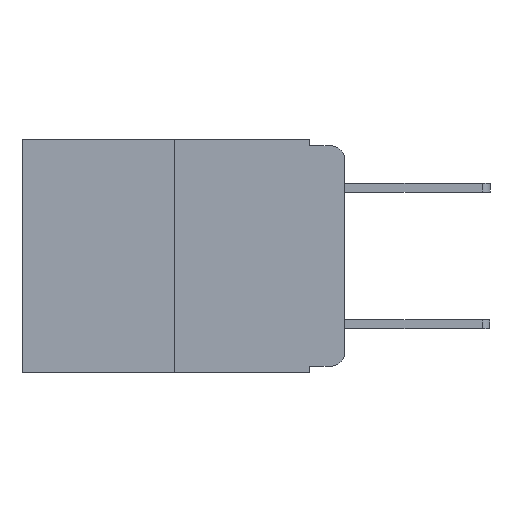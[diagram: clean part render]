
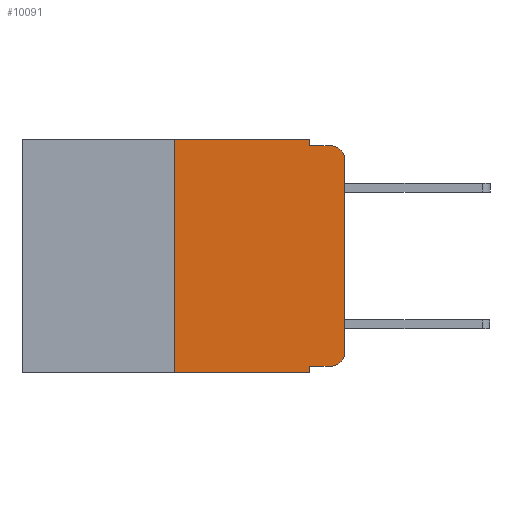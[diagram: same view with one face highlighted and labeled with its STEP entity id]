
A CAD part, left-side view. The second image highlights one B-rep face of the part: STEP entity #10091.
In plain terms, the highlighted planar face has unit normal (-1, 0, 0).
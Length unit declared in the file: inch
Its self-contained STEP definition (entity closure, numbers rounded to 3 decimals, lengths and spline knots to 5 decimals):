
#117 = ORIENTED_EDGE ( 'NONE', *, *, #6094, .T. ) ;
#219 = CARTESIAN_POINT ( 'NONE',  ( 0., 0.473, -0.343 ) ) ;
#726 = EDGE_CURVE ( 'NONE', #4347, #4538, #12148, .T. ) ;
#972 = DIRECTION ( 'NONE',  ( 1., 0., 0. ) ) ;
#1107 = VERTEX_POINT ( 'NONE', #7958 ) ;
#1331 = VERTEX_POINT ( 'NONE', #15850 ) ;
#1384 = DIRECTION ( 'NONE',  ( 0., 0., -1. ) ) ;
#1502 = DIRECTION ( 'NONE',  ( -1., 0., 0. ) ) ;
#1890 = ORIENTED_EDGE ( 'NONE', *, *, #19439, .T. ) ;
#1897 = EDGE_LOOP ( 'NONE', ( #117, #9946, #16369, #5119, #18560, #11007, #1890, #16342, #3068, #16850 ) ) ;
#2301 = VERTEX_POINT ( 'NONE', #17408 ) ;
#2786 = EDGE_CURVE ( 'NONE', #1331, #1107, #20935, .T. ) ;
#2883 = VECTOR ( 'NONE', #16946, 39.37008 ) ;
#3055 = CARTESIAN_POINT ( 'NONE',  ( 0., 0.473, 0. ) ) ;
#3068 = ORIENTED_EDGE ( 'NONE', *, *, #2786, .T. ) ;
#3369 = VECTOR ( 'NONE', #11215, 39.37008 ) ;
#3531 = CARTESIAN_POINT ( 'NONE',  ( 0., 0.02, -0.03 ) ) ;
#3875 = CIRCLE ( 'NONE', #17647, 0.02 ) ;
#4264 = CARTESIAN_POINT ( 'NONE',  ( 0., 0., -0.313 ) ) ;
#4347 = VERTEX_POINT ( 'NONE', #21938 ) ;
#4538 = VERTEX_POINT ( 'NONE', #9941 ) ;
#5119 = ORIENTED_EDGE ( 'NONE', *, *, #13500, .F. ) ;
#5475 = VECTOR ( 'NONE', #10614, 39.37008 ) ;
#5913 = EDGE_CURVE ( 'NONE', #1331, #17348, #18840, .T. ) ;
#6094 = EDGE_CURVE ( 'NONE', #14765, #4347, #20506, .T. ) ;
#6345 = AXIS2_PLACEMENT_3D ( 'NONE', #16681, #972, #13532 ) ;
#6657 = VECTOR ( 'NONE', #13686, 39.37008 ) ;
#7042 = LINE ( 'NONE', #16831, #15542 ) ;
#7115 = CARTESIAN_POINT ( 'NONE',  ( 0., 0.051, -0.333 ) ) ;
#7448 = VECTOR ( 'NONE', #18966, 39.37008 ) ;
#7713 = EDGE_CURVE ( 'NONE', #11179, #2301, #16749, .T. ) ;
#7958 = CARTESIAN_POINT ( 'NONE',  ( 0., 0.02, -0.333 ) ) ;
#8108 = VERTEX_POINT ( 'NONE', #9652 ) ;
#8570 = CARTESIAN_POINT ( 'NONE',  ( 0., 0.051, -0.343 ) ) ;
#8830 = CARTESIAN_POINT ( 'NONE',  ( 0., 0.051, 0. ) ) ;
#8865 = EDGE_CURVE ( 'NONE', #2301, #18205, #12433, .T. ) ;
#9652 = CARTESIAN_POINT ( 'NONE',  ( 0., 0.051, -0.01 ) ) ;
#9783 = EDGE_CURVE ( 'NONE', #8108, #4538, #15671, .T. ) ;
#9941 = CARTESIAN_POINT ( 'NONE',  ( 0., 0.02, -0.01 ) ) ;
#9946 = ORIENTED_EDGE ( 'NONE', *, *, #726, .T. ) ;
#9983 = DIRECTION ( 'NONE',  ( -1., 0., 0. ) ) ;
#10091 = ADVANCED_FACE ( 'NONE', ( #18146 ), #21343, .F. ) ;
#10614 = DIRECTION ( 'NONE',  ( 0., 0., -1. ) ) ;
#11007 = ORIENTED_EDGE ( 'NONE', *, *, #7713, .F. ) ;
#11179 = VERTEX_POINT ( 'NONE', #16640 ) ;
#11215 = DIRECTION ( 'NONE',  ( 0., -1., 0. ) ) ;
#11993 = CARTESIAN_POINT ( 'NONE',  ( 0., 0.051, -0.01 ) ) ;
#12148 = CIRCLE ( 'NONE', #12987, 0.02 ) ;
#12433 = LINE ( 'NONE', #3055, #2883 ) ;
#12499 = VECTOR ( 'NONE', #19750, 39.37008 ) ;
#12582 = VECTOR ( 'NONE', #18663, 39.37008 ) ;
#12755 = EDGE_CURVE ( 'NONE', #1107, #14765, #3875, .T. ) ;
#12987 = AXIS2_PLACEMENT_3D ( 'NONE', #3531, #1502, #1384 ) ;
#13500 = EDGE_CURVE ( 'NONE', #18205, #8108, #7042, .T. ) ;
#13532 = DIRECTION ( 'NONE',  ( 0., 0., -1. ) ) ;
#13686 = DIRECTION ( 'NONE',  ( 0., -1., 0. ) ) ;
#14765 = VERTEX_POINT ( 'NONE', #4264 ) ;
#15070 = CARTESIAN_POINT ( 'NONE',  ( 0., 0.25, 0. ) ) ;
#15542 = VECTOR ( 'NONE', #16764, 39.37008 ) ;
#15671 = LINE ( 'NONE', #11993, #6657 ) ;
#15811 = CARTESIAN_POINT ( 'NONE',  ( 0., 0., 0. ) ) ;
#15850 = CARTESIAN_POINT ( 'NONE',  ( 0., 0.051, -0.333 ) ) ;
#16342 = ORIENTED_EDGE ( 'NONE', *, *, #5913, .F. ) ;
#16369 = ORIENTED_EDGE ( 'NONE', *, *, #9783, .F. ) ;
#16640 = CARTESIAN_POINT ( 'NONE',  ( 0., 0.25, -0.343 ) ) ;
#16681 = CARTESIAN_POINT ( 'NONE',  ( 0., 0.473, 0. ) ) ;
#16749 = LINE ( 'NONE', #15070, #12499 ) ;
#16764 = DIRECTION ( 'NONE',  ( 0., 0., -1. ) ) ;
#16831 = CARTESIAN_POINT ( 'NONE',  ( 0., 0.051, 0. ) ) ;
#16850 = ORIENTED_EDGE ( 'NONE', *, *, #12755, .T. ) ;
#16946 = DIRECTION ( 'NONE',  ( 0., -1., 0. ) ) ;
#17348 = VERTEX_POINT ( 'NONE', #8570 ) ;
#17408 = CARTESIAN_POINT ( 'NONE',  ( 0., 0.25, 0. ) ) ;
#17647 = AXIS2_PLACEMENT_3D ( 'NONE', #19633, #9983, #21195 ) ;
#18146 = FACE_OUTER_BOUND ( 'NONE', #1897, .T. ) ;
#18205 = VERTEX_POINT ( 'NONE', #18350 ) ;
#18350 = CARTESIAN_POINT ( 'NONE',  ( 0., 0.051, 0. ) ) ;
#18560 = ORIENTED_EDGE ( 'NONE', *, *, #8865, .F. ) ;
#18663 = DIRECTION ( 'NONE',  ( 0., -1., 0. ) ) ;
#18840 = LINE ( 'NONE', #8830, #5475 ) ;
#18966 = DIRECTION ( 'NONE',  ( 0., 0., 1. ) ) ;
#19439 = EDGE_CURVE ( 'NONE', #11179, #17348, #20717, .T. ) ;
#19633 = CARTESIAN_POINT ( 'NONE',  ( 0., 0.02, -0.313 ) ) ;
#19750 = DIRECTION ( 'NONE',  ( 0., 0., 1. ) ) ;
#20506 = LINE ( 'NONE', #15811, #7448 ) ;
#20717 = LINE ( 'NONE', #219, #3369 ) ;
#20935 = LINE ( 'NONE', #7115, #12582 ) ;
#21195 = DIRECTION ( 'NONE',  ( 0., 0., -1. ) ) ;
#21343 = PLANE ( 'NONE',  #6345 ) ;
#21938 = CARTESIAN_POINT ( 'NONE',  ( 0., 0., -0.03 ) ) ;
